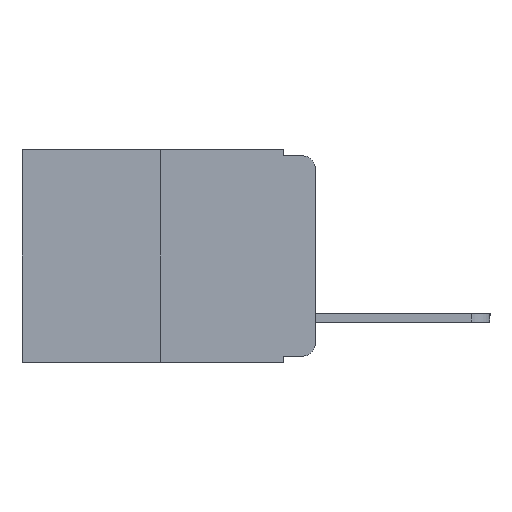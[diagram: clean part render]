
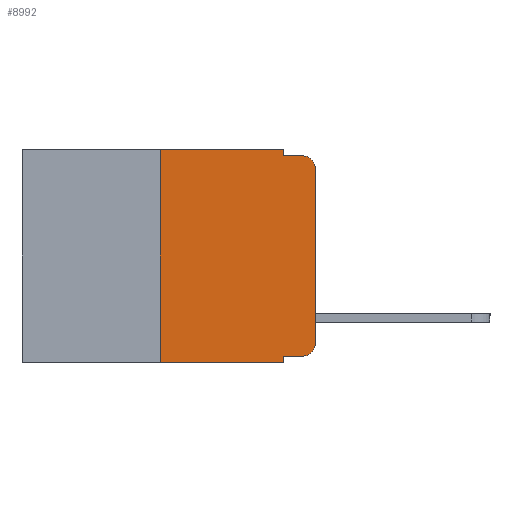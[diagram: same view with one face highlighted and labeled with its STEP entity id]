
A CAD part, left-side view. The second image highlights one B-rep face of the part: STEP entity #8992.
In plain terms, the highlighted planar face has unit normal (-1, 0, 0).
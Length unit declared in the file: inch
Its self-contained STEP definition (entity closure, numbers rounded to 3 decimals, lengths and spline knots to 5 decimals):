
#173 = EDGE_CURVE ( 'NONE', #3969, #17751, #8815, .T. ) ;
#309 = VERTEX_POINT ( 'NONE', #11909 ) ;
#481 = FACE_OUTER_BOUND ( 'NONE', #5600, .T. ) ;
#590 = VERTEX_POINT ( 'NONE', #12478 ) ;
#1242 = EDGE_CURVE ( 'NONE', #590, #17751, #5747, .T. ) ;
#1479 = DIRECTION ( 'NONE',  ( 0., -1., 0. ) ) ;
#1568 = CARTESIAN_POINT ( 'NONE',  ( 0., 0.473, -0.343 ) ) ;
#1972 = CARTESIAN_POINT ( 'NONE',  ( 0., 0.051, -0.343 ) ) ;
#2332 = EDGE_CURVE ( 'NONE', #6681, #590, #7823, .T. ) ;
#3147 = DIRECTION ( 'NONE',  ( 0., 0., -1. ) ) ;
#3929 = EDGE_CURVE ( 'NONE', #5087, #14762, #5835, .T. ) ;
#3950 = VECTOR ( 'NONE', #10144, 39.37008 ) ;
#3969 = VERTEX_POINT ( 'NONE', #16657 ) ;
#4083 = CARTESIAN_POINT ( 'NONE',  ( 0., 0.473, 0. ) ) ;
#4498 = ORIENTED_EDGE ( 'NONE', *, *, #3929, .T. ) ;
#5087 = VERTEX_POINT ( 'NONE', #16102 ) ;
#5600 = EDGE_LOOP ( 'NONE', ( #8058, #15472, #14836, #16679, #9450, #11366, #4498, #7537, #14723, #14064 ) ) ;
#5689 = LINE ( 'NONE', #13952, #16329 ) ;
#5747 = CIRCLE ( 'NONE', #15762, 0.02 ) ;
#5835 = LINE ( 'NONE', #1568, #9453 ) ;
#6681 = VERTEX_POINT ( 'NONE', #16680 ) ;
#6819 = CARTESIAN_POINT ( 'NONE',  ( 0., 0.051, 0. ) ) ;
#6829 = CARTESIAN_POINT ( 'NONE',  ( 0., 0.02, -0.313 ) ) ;
#7346 = LINE ( 'NONE', #9330, #14029 ) ;
#7417 = CARTESIAN_POINT ( 'NONE',  ( 0., 0.25, 0. ) ) ;
#7537 = ORIENTED_EDGE ( 'NONE', *, *, #15387, .F. ) ;
#7594 = LINE ( 'NONE', #7417, #3950 ) ;
#7666 = VERTEX_POINT ( 'NONE', #6819 ) ;
#7823 = LINE ( 'NONE', #10957, #17179 ) ;
#8058 = ORIENTED_EDGE ( 'NONE', *, *, #2332, .T. ) ;
#8209 = DIRECTION ( 'NONE',  ( 0., 0., -1. ) ) ;
#8549 = CARTESIAN_POINT ( 'NONE',  ( 0., 0.051, -0.333 ) ) ;
#8613 = DIRECTION ( 'NONE',  ( 0., -1., 0. ) ) ;
#8815 = LINE ( 'NONE', #13571, #11904 ) ;
#8992 = ADVANCED_FACE ( 'NONE', ( #481 ), #16147, .F. ) ;
#9330 = CARTESIAN_POINT ( 'NONE',  ( 0., 0.051, 0. ) ) ;
#9450 = ORIENTED_EDGE ( 'NONE', *, *, #16173, .F. ) ;
#9453 = VECTOR ( 'NONE', #8613, 39.37008 ) ;
#9580 = DIRECTION ( 'NONE',  ( 0., 0., -1. ) ) ;
#10144 = DIRECTION ( 'NONE',  ( 0., 0., 1. ) ) ;
#10957 = CARTESIAN_POINT ( 'NONE',  ( 0., 0., 0. ) ) ;
#11279 = DIRECTION ( 'NONE',  ( 0., -1., 0. ) ) ;
#11297 = CARTESIAN_POINT ( 'NONE',  ( 0., 0.051, 0. ) ) ;
#11366 = ORIENTED_EDGE ( 'NONE', *, *, #16272, .F. ) ;
#11904 = VECTOR ( 'NONE', #13074, 39.37008 ) ;
#11909 = CARTESIAN_POINT ( 'NONE',  ( 0., 0.25, 0. ) ) ;
#11964 = DIRECTION ( 'NONE',  ( 0., 0., -1. ) ) ;
#12031 = VECTOR ( 'NONE', #1479, 39.37008 ) ;
#12478 = CARTESIAN_POINT ( 'NONE',  ( 0., 0., -0.03 ) ) ;
#12630 = DIRECTION ( 'NONE',  ( 0., 0., 1. ) ) ;
#12634 = VECTOR ( 'NONE', #3147, 39.37008 ) ;
#12800 = CIRCLE ( 'NONE', #15149, 0.02 ) ;
#13036 = VERTEX_POINT ( 'NONE', #13744 ) ;
#13074 = DIRECTION ( 'NONE',  ( 0., -1., 0. ) ) ;
#13571 = CARTESIAN_POINT ( 'NONE',  ( 0., 0.051, -0.01 ) ) ;
#13621 = EDGE_CURVE ( 'NONE', #15737, #6681, #12800, .T. ) ;
#13744 = CARTESIAN_POINT ( 'NONE',  ( 0., 0.051, -0.333 ) ) ;
#13952 = CARTESIAN_POINT ( 'NONE',  ( 0., 0.473, 0. ) ) ;
#14029 = VECTOR ( 'NONE', #11964, 39.37008 ) ;
#14064 = ORIENTED_EDGE ( 'NONE', *, *, #13621, .T. ) ;
#14423 = CARTESIAN_POINT ( 'NONE',  ( 0., 0.02, -0.03 ) ) ;
#14484 = DIRECTION ( 'NONE',  ( 0., 0., -1. ) ) ;
#14505 = EDGE_CURVE ( 'NONE', #13036, #15737, #15545, .T. ) ;
#14543 = DIRECTION ( 'NONE',  ( -1., 0., 0. ) ) ;
#14723 = ORIENTED_EDGE ( 'NONE', *, *, #14505, .T. ) ;
#14762 = VERTEX_POINT ( 'NONE', #1972 ) ;
#14836 = ORIENTED_EDGE ( 'NONE', *, *, #173, .F. ) ;
#14918 = LINE ( 'NONE', #11297, #12634 ) ;
#15105 = AXIS2_PLACEMENT_3D ( 'NONE', #4083, #17504, #9580 ) ;
#15149 = AXIS2_PLACEMENT_3D ( 'NONE', #6829, #16141, #8209 ) ;
#15387 = EDGE_CURVE ( 'NONE', #13036, #14762, #14918, .T. ) ;
#15472 = ORIENTED_EDGE ( 'NONE', *, *, #1242, .T. ) ;
#15545 = LINE ( 'NONE', #8549, #12031 ) ;
#15737 = VERTEX_POINT ( 'NONE', #15800 ) ;
#15762 = AXIS2_PLACEMENT_3D ( 'NONE', #14423, #14543, #14484 ) ;
#15800 = CARTESIAN_POINT ( 'NONE',  ( 0., 0.02, -0.333 ) ) ;
#16102 = CARTESIAN_POINT ( 'NONE',  ( 0., 0.25, -0.343 ) ) ;
#16141 = DIRECTION ( 'NONE',  ( -1., 0., 0. ) ) ;
#16147 = PLANE ( 'NONE',  #15105 ) ;
#16173 = EDGE_CURVE ( 'NONE', #309, #7666, #5689, .T. ) ;
#16272 = EDGE_CURVE ( 'NONE', #5087, #309, #7594, .T. ) ;
#16329 = VECTOR ( 'NONE', #11279, 39.37008 ) ;
#16657 = CARTESIAN_POINT ( 'NONE',  ( 0., 0.051, -0.01 ) ) ;
#16679 = ORIENTED_EDGE ( 'NONE', *, *, #17183, .F. ) ;
#16680 = CARTESIAN_POINT ( 'NONE',  ( 0., 0., -0.313 ) ) ;
#16877 = CARTESIAN_POINT ( 'NONE',  ( 0., 0.02, -0.01 ) ) ;
#17179 = VECTOR ( 'NONE', #12630, 39.37008 ) ;
#17183 = EDGE_CURVE ( 'NONE', #7666, #3969, #7346, .T. ) ;
#17504 = DIRECTION ( 'NONE',  ( 1., 0., 0. ) ) ;
#17751 = VERTEX_POINT ( 'NONE', #16877 ) ;
